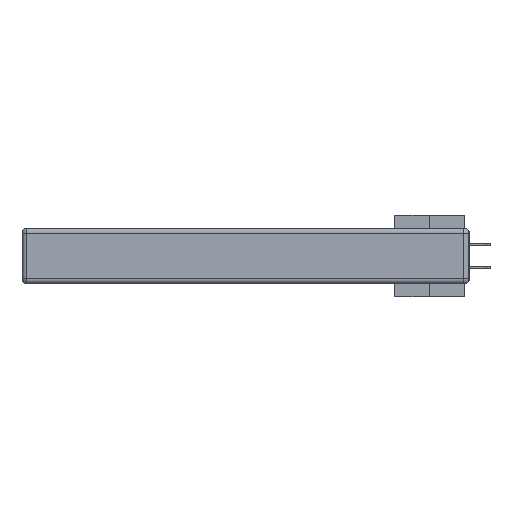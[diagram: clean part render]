
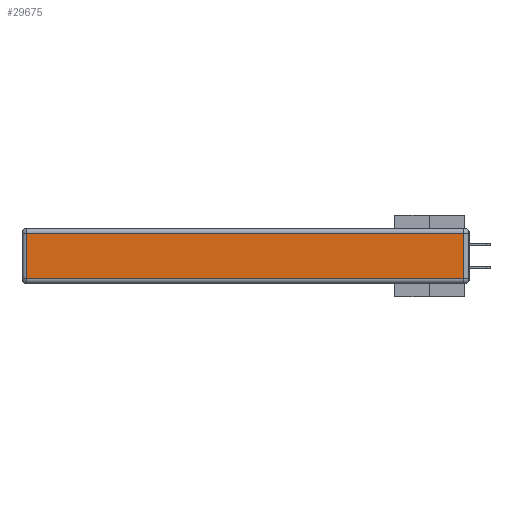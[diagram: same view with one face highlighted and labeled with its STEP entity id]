
A CAD part, left-side view. The second image highlights one B-rep face of the part: STEP entity #29675.
In plain terms, the highlighted planar face has unit normal (-1, 0, 0).
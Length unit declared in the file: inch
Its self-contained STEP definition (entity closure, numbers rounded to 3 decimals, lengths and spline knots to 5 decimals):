
#1332 = LINE ( 'NONE', #3923, #34425 ) ;
#2498 = LINE ( 'NONE', #4975, #22996 ) ;
#2816 = LINE ( 'NONE', #3688, #30456 ) ;
#3280 = VECTOR ( 'NONE', #12920, 39.37008 ) ;
#3688 = CARTESIAN_POINT ( 'NONE',  ( 0., 2.72, -0.343 ) ) ;
#3923 = CARTESIAN_POINT ( 'NONE',  ( 0., 0., -0.313 ) ) ;
#3956 = PLANE ( 'NONE',  #18931 ) ;
#4955 = CARTESIAN_POINT ( 'NONE',  ( 0., 0.03, -0.343 ) ) ;
#4975 = CARTESIAN_POINT ( 'NONE',  ( 0., 2.75, -0.03 ) ) ;
#5629 = ORIENTED_EDGE ( 'NONE', *, *, #33406, .T. ) ;
#8981 = CARTESIAN_POINT ( 'NONE',  ( 0., 2.72, -0.03 ) ) ;
#10339 = EDGE_CURVE ( 'NONE', #26993, #24194, #1332, .T. ) ;
#10408 = LINE ( 'NONE', #4955, #3280 ) ;
#11533 = VERTEX_POINT ( 'NONE', #27611 ) ;
#11922 = DIRECTION ( 'NONE',  ( -1., 0., 0. ) ) ;
#12439 = EDGE_CURVE ( 'NONE', #11533, #30186, #2498, .T. ) ;
#12801 = ORIENTED_EDGE ( 'NONE', *, *, #12439, .T. ) ;
#12920 = DIRECTION ( 'NONE',  ( 0., 0., 1. ) ) ;
#13431 = ORIENTED_EDGE ( 'NONE', *, *, #10339, .T. ) ;
#13769 = EDGE_CURVE ( 'NONE', #30186, #26993, #2816, .T. ) ;
#14575 = DIRECTION ( 'NONE',  ( 0., -1., 0. ) ) ;
#18931 = AXIS2_PLACEMENT_3D ( 'NONE', #22217, #11922, #22550 ) ;
#20163 = EDGE_LOOP ( 'NONE', ( #13431, #5629, #12801, #33305 ) ) ;
#22217 = CARTESIAN_POINT ( 'NONE',  ( 0., 0., -0.343 ) ) ;
#22550 = DIRECTION ( 'NONE',  ( 0., 0., 1. ) ) ;
#22996 = VECTOR ( 'NONE', #31553, 39.37008 ) ;
#24194 = VERTEX_POINT ( 'NONE', #28861 ) ;
#26993 = VERTEX_POINT ( 'NONE', #34197 ) ;
#27611 = CARTESIAN_POINT ( 'NONE',  ( 0., 0.03, -0.03 ) ) ;
#28005 = DIRECTION ( 'NONE',  ( 0., 0., -1. ) ) ;
#28861 = CARTESIAN_POINT ( 'NONE',  ( 0., 0.03, -0.313 ) ) ;
#29675 = ADVANCED_FACE ( 'NONE', ( #32826 ), #3956, .T. ) ;
#30186 = VERTEX_POINT ( 'NONE', #8981 ) ;
#30456 = VECTOR ( 'NONE', #28005, 39.37008 ) ;
#31553 = DIRECTION ( 'NONE',  ( 0., 1., 0. ) ) ;
#32826 = FACE_OUTER_BOUND ( 'NONE', #20163, .T. ) ;
#33305 = ORIENTED_EDGE ( 'NONE', *, *, #13769, .T. ) ;
#33406 = EDGE_CURVE ( 'NONE', #24194, #11533, #10408, .T. ) ;
#34197 = CARTESIAN_POINT ( 'NONE',  ( 0., 2.72, -0.313 ) ) ;
#34425 = VECTOR ( 'NONE', #14575, 39.37008 ) ;
